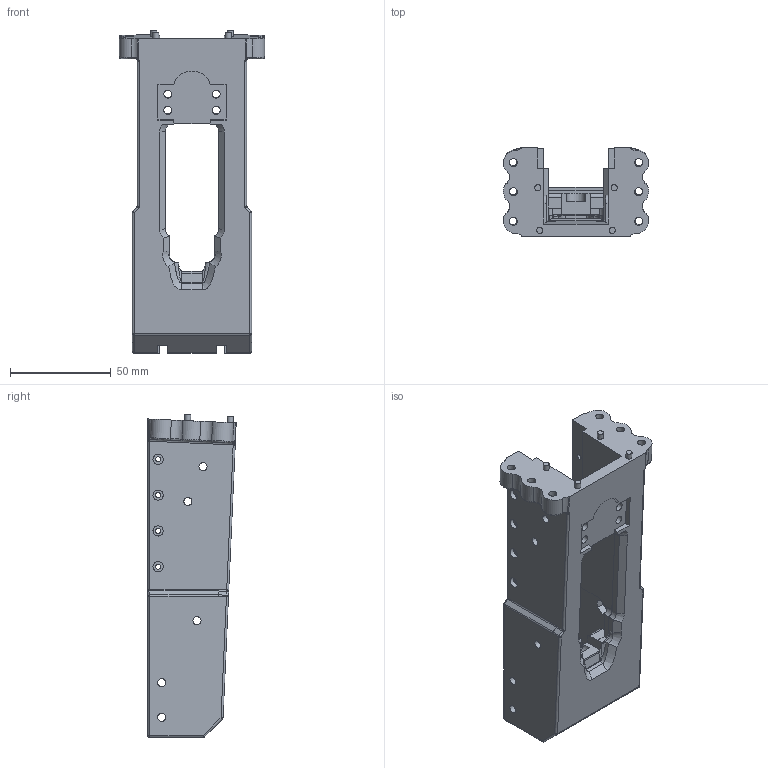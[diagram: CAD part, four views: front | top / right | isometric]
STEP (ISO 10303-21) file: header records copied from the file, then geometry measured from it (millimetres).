
FILE_DESCRIPTION(/* description */ (''),/* implementation_level */ '2;1');
FILE_NAME(/* name */ 'Plastikov v1.0 Front Receiver.stp',/* time_stamp */ '2020-05-01T15:29:55-05:00',/* author */ ('johne'),/* organization */ (''),/* preprocessor_version */ 'ST-DEVELOPER v18',/* originating_system */ 'Autodesk Inventor 2020',/* authorisation */ '');
FILE_SCHEMA (('AUTOMOTIVE_DESIGN { 1 0 10303 214 3 1 1 }'));
Length unit declared in the file: millimetre
Products named in the file (1): Plastikov v0.9 Front Receiver
Bounding box: 72.2 x 43.88 x 160.38 mm (x, y, z)
Volume: 187011.1 mm3; surface area: 45576.2 mm2
Topology: 1 solids, 1 shells, 358 faces, 931 edges, 587 vertices
Faces by surface type: plane 173, cylinder 111, bspline 39, torus 16, sphere 13, cone 6
Full cylindrical faces by diameter (mm): 2.5 x8, 3 x4, 4 x21, 4.05 x1, 5.08 x8
Entity records: 12259 total; most frequent: CARTESIAN_POINT 3334, ORIENTED_EDGE 1846, DIRECTION 1830, EDGE_CURVE 923, AXIS2_PLACEMENT_3D 640, VERTEX_POINT 587, LINE 550, VECTOR 550
